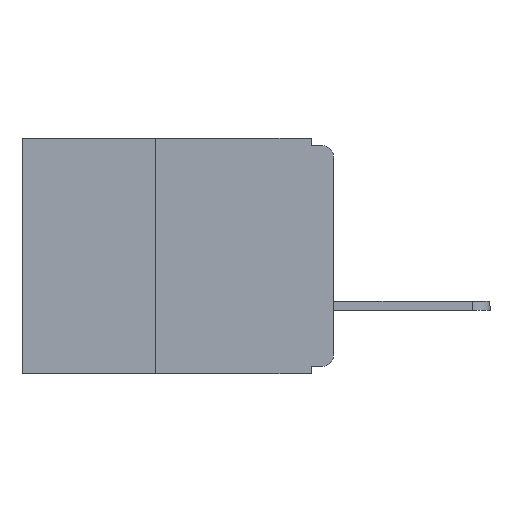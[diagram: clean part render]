
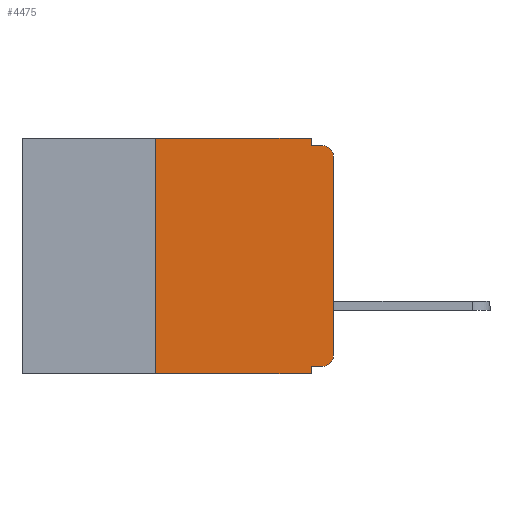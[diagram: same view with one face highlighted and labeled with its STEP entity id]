
A CAD part, left-side view. The second image highlights one B-rep face of the part: STEP entity #4475.
In plain terms, the highlighted planar face has unit normal (-1, 0, 0).
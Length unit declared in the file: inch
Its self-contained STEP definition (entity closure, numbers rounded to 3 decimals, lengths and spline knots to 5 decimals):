
#90 = EDGE_CURVE ( 'NONE', #17643, #16195, #6698, .T. ) ;
#1060 = CARTESIAN_POINT ( 'NONE',  ( 0., 0.25, -0.33 ) ) ;
#1226 = ORIENTED_EDGE ( 'NONE', *, *, #23900, .F. ) ;
#1449 = EDGE_CURVE ( 'NONE', #11047, #4731, #25938, .T. ) ;
#1714 = EDGE_CURVE ( 'NONE', #9563, #21381, #24942, .T. ) ;
#2105 = EDGE_CURVE ( 'NONE', #9563, #17643, #3235, .T. ) ;
#2198 = VERTEX_POINT ( 'NONE', #7371 ) ;
#2921 = CARTESIAN_POINT ( 'NONE',  ( 0., 0.015, -0.32 ) ) ;
#3235 = LINE ( 'NONE', #8673, #25575 ) ;
#3447 = LINE ( 'NONE', #12469, #25136 ) ;
#3774 = VECTOR ( 'NONE', #13472, 39.37008 ) ;
#3906 = CARTESIAN_POINT ( 'NONE',  ( 0., 0.031, -0.33 ) ) ;
#3921 = DIRECTION ( 'NONE',  ( 0., -1., 0. ) ) ;
#4136 = VECTOR ( 'NONE', #21373, 39.37008 ) ;
#4229 = ORIENTED_EDGE ( 'NONE', *, *, #90, .F. ) ;
#4358 = VERTEX_POINT ( 'NONE', #11803 ) ;
#4436 = CARTESIAN_POINT ( 'NONE',  ( 0., 0., -0.025 ) ) ;
#4475 = ADVANCED_FACE ( 'NONE', ( #21451 ), #18662, .F. ) ;
#4731 = VERTEX_POINT ( 'NONE', #23848 ) ;
#5983 = ORIENTED_EDGE ( 'NONE', *, *, #18825, .T. ) ;
#6229 = DIRECTION ( 'NONE',  ( 0., 0., -1. ) ) ;
#6422 = CARTESIAN_POINT ( 'NONE',  ( 0., 0.437, 0. ) ) ;
#6460 = AXIS2_PLACEMENT_3D ( 'NONE', #18903, #14983, #25713 ) ;
#6698 = LINE ( 'NONE', #25282, #23291 ) ;
#6702 = ORIENTED_EDGE ( 'NONE', *, *, #2105, .F. ) ;
#7371 = CARTESIAN_POINT ( 'NONE',  ( 0., 0.25, 0. ) ) ;
#7688 = EDGE_LOOP ( 'NONE', ( #17372, #18539, #1226, #18679, #26111, #17637, #5983, #4229, #6702, #16141 ) ) ;
#8673 = CARTESIAN_POINT ( 'NONE',  ( 0., 0., -0.32 ) ) ;
#8980 = CARTESIAN_POINT ( 'NONE',  ( 0., 0.031, 0. ) ) ;
#9537 = LINE ( 'NONE', #24236, #3774 ) ;
#9563 = VERTEX_POINT ( 'NONE', #2921 ) ;
#9578 = LINE ( 'NONE', #27182, #21071 ) ;
#9882 = LINE ( 'NONE', #10520, #4136 ) ;
#9901 = AXIS2_PLACEMENT_3D ( 'NONE', #24995, #24964, #6229 ) ;
#10027 = DIRECTION ( 'NONE',  ( 1., 0., 0. ) ) ;
#10520 = CARTESIAN_POINT ( 'NONE',  ( 0., 0.437, -0.33 ) ) ;
#11028 = CARTESIAN_POINT ( 'NONE',  ( 0., 0.031, -0.32 ) ) ;
#11047 = VERTEX_POINT ( 'NONE', #4436 ) ;
#11141 = EDGE_CURVE ( 'NONE', #11898, #4358, #27160, .T. ) ;
#11354 = EDGE_CURVE ( 'NONE', #15632, #2198, #9578, .T. ) ;
#11803 = CARTESIAN_POINT ( 'NONE',  ( 0., 0.031, -0.01 ) ) ;
#11898 = VERTEX_POINT ( 'NONE', #18297 ) ;
#12469 = CARTESIAN_POINT ( 'NONE',  ( 0., 0., -0.01 ) ) ;
#13472 = DIRECTION ( 'NONE',  ( 0., 0., 1. ) ) ;
#14064 = LINE ( 'NONE', #6422, #19811 ) ;
#14239 = DIRECTION ( 'NONE',  ( 0., 0., 1. ) ) ;
#14983 = DIRECTION ( 'NONE',  ( -1., 0., 0. ) ) ;
#14993 = VECTOR ( 'NONE', #22099, 39.37008 ) ;
#15632 = VERTEX_POINT ( 'NONE', #1060 ) ;
#16141 = ORIENTED_EDGE ( 'NONE', *, *, #1714, .T. ) ;
#16195 = VERTEX_POINT ( 'NONE', #3906 ) ;
#16906 = EDGE_CURVE ( 'NONE', #2198, #11898, #14064, .T. ) ;
#17372 = ORIENTED_EDGE ( 'NONE', *, *, #19050, .T. ) ;
#17637 = ORIENTED_EDGE ( 'NONE', *, *, #11354, .F. ) ;
#17643 = VERTEX_POINT ( 'NONE', #11028 ) ;
#18297 = CARTESIAN_POINT ( 'NONE',  ( 0., 0.031, 0. ) ) ;
#18539 = ORIENTED_EDGE ( 'NONE', *, *, #1449, .T. ) ;
#18662 = PLANE ( 'NONE',  #19025 ) ;
#18679 = ORIENTED_EDGE ( 'NONE', *, *, #11141, .F. ) ;
#18825 = EDGE_CURVE ( 'NONE', #15632, #16195, #9882, .T. ) ;
#18903 = CARTESIAN_POINT ( 'NONE',  ( 0., 0.015, -0.305 ) ) ;
#19025 = AXIS2_PLACEMENT_3D ( 'NONE', #25100, #10027, #25185 ) ;
#19050 = EDGE_CURVE ( 'NONE', #21381, #11047, #9537, .T. ) ;
#19466 = DIRECTION ( 'NONE',  ( 0., 1., 0. ) ) ;
#19811 = VECTOR ( 'NONE', #23750, 39.37008 ) ;
#21071 = VECTOR ( 'NONE', #14239, 39.37008 ) ;
#21373 = DIRECTION ( 'NONE',  ( 0., -1., 0. ) ) ;
#21381 = VERTEX_POINT ( 'NONE', #23933 ) ;
#21451 = FACE_OUTER_BOUND ( 'NONE', #7688, .T. ) ;
#22099 = DIRECTION ( 'NONE',  ( 0., 0., -1. ) ) ;
#23291 = VECTOR ( 'NONE', #24855, 39.37008 ) ;
#23750 = DIRECTION ( 'NONE',  ( 0., -1., 0. ) ) ;
#23848 = CARTESIAN_POINT ( 'NONE',  ( 0., 0.015, -0.01 ) ) ;
#23900 = EDGE_CURVE ( 'NONE', #4358, #4731, #3447, .T. ) ;
#23933 = CARTESIAN_POINT ( 'NONE',  ( 0., 0., -0.305 ) ) ;
#24236 = CARTESIAN_POINT ( 'NONE',  ( 0., 0., 0. ) ) ;
#24855 = DIRECTION ( 'NONE',  ( 0., 0., -1. ) ) ;
#24942 = CIRCLE ( 'NONE', #6460, 0.015 ) ;
#24964 = DIRECTION ( 'NONE',  ( -1., 0., 0. ) ) ;
#24995 = CARTESIAN_POINT ( 'NONE',  ( 0., 0.015, -0.025 ) ) ;
#25100 = CARTESIAN_POINT ( 'NONE',  ( 0., 0.437, 0. ) ) ;
#25136 = VECTOR ( 'NONE', #3921, 39.37008 ) ;
#25185 = DIRECTION ( 'NONE',  ( 0., 0., -1. ) ) ;
#25282 = CARTESIAN_POINT ( 'NONE',  ( 0., 0.031, -0.33 ) ) ;
#25575 = VECTOR ( 'NONE', #19466, 39.37008 ) ;
#25713 = DIRECTION ( 'NONE',  ( 0., 0., -1. ) ) ;
#25938 = CIRCLE ( 'NONE', #9901, 0.015 ) ;
#26111 = ORIENTED_EDGE ( 'NONE', *, *, #16906, .F. ) ;
#27160 = LINE ( 'NONE', #8980, #14993 ) ;
#27182 = CARTESIAN_POINT ( 'NONE',  ( 0., 0.25, -0.33 ) ) ;
